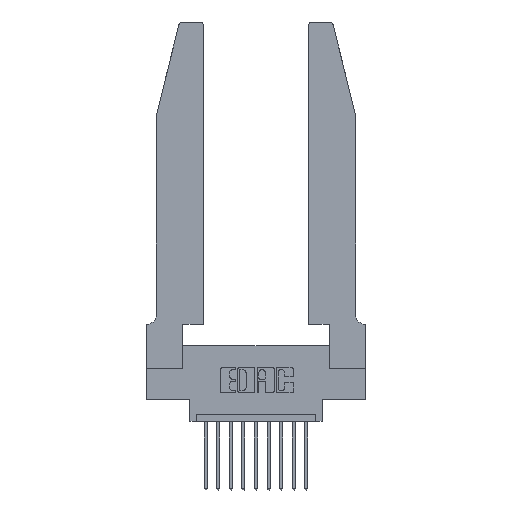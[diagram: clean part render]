
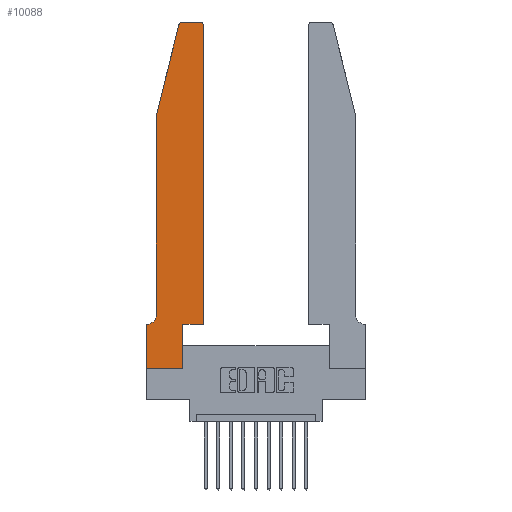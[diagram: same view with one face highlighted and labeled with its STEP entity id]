
A CAD part, top view. The second image highlights one B-rep face of the part: STEP entity #10088.
In plain terms, the highlighted planar face has unit normal (0, 0, 1).
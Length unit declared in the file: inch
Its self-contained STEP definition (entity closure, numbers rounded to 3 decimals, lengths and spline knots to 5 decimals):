
#271 = AXIS2_PLACEMENT_3D ( 'NONE', #14852, #7218, #7381 ) ;
#731 = DIRECTION ( 'NONE',  ( 1., 0., 0. ) ) ;
#881 = ORIENTED_EDGE ( 'NONE', *, *, #12736, .T. ) ;
#1047 = ORIENTED_EDGE ( 'NONE', *, *, #1208, .T. ) ;
#1116 = VECTOR ( 'NONE', #6995, 39.37008 ) ;
#1201 = VECTOR ( 'NONE', #15198, 39.37008 ) ;
#1208 = EDGE_CURVE ( 'NONE', #14253, #4587, #13218, .T. ) ;
#1744 = CARTESIAN_POINT ( 'NONE',  ( 0.0755, 2., 0.37 ) ) ;
#1786 = CARTESIAN_POINT ( 'NONE',  ( 0.2865, 0., 0.37 ) ) ;
#1848 = EDGE_CURVE ( 'NONE', #2867, #7956, #15561, .T. ) ;
#1938 = ORIENTED_EDGE ( 'NONE', *, *, #12678, .T. ) ;
#2620 = CARTESIAN_POINT ( 'NONE',  ( 0.4205, 2.75, 0.37 ) ) ;
#2723 = FACE_OUTER_BOUND ( 'NONE', #6679, .T. ) ;
#2867 = VERTEX_POINT ( 'NONE', #9042 ) ;
#2932 = ORIENTED_EDGE ( 'NONE', *, *, #13490, .T. ) ;
#2975 = LINE ( 'NONE', #7670, #1201 ) ;
#2981 = EDGE_CURVE ( 'NONE', #8498, #5443, #2975, .T. ) ;
#2985 = CARTESIAN_POINT ( 'NONE',  ( 0., 0., 0.37 ) ) ;
#3156 = CARTESIAN_POINT ( 'NONE',  ( 0., 0., 0.37 ) ) ;
#3195 = DIRECTION ( 'NONE',  ( 0., -1., 0. ) ) ;
#3352 = ORIENTED_EDGE ( 'NONE', *, *, #4293, .T. ) ;
#3621 = CARTESIAN_POINT ( 'NONE',  ( 0.2865, 0.35, 0.37 ) ) ;
#3913 = AXIS2_PLACEMENT_3D ( 'NONE', #9033, #8985, #4082 ) ;
#3989 = CARTESIAN_POINT ( 'NONE',  ( 0.2605, 2.75, 0.37 ) ) ;
#4014 = ORIENTED_EDGE ( 'NONE', *, *, #2981, .T. ) ;
#4082 = DIRECTION ( 'NONE',  ( -1., 0., 0. ) ) ;
#4103 = ORIENTED_EDGE ( 'NONE', *, *, #10048, .T. ) ;
#4210 = VECTOR ( 'NONE', #16006, 39.37008 ) ;
#4254 = DIRECTION ( 'NONE',  ( -0.239, -0.971, 0. ) ) ;
#4293 = EDGE_CURVE ( 'NONE', #6805, #8498, #6608, .T. ) ;
#4323 = CARTESIAN_POINT ( 'NONE',  ( 0., 0., 0.37 ) ) ;
#4379 = DIRECTION ( 'NONE',  ( 1., 0., 0. ) ) ;
#4436 = CIRCLE ( 'NONE', #271, 0.03 ) ;
#4440 = VERTEX_POINT ( 'NONE', #13590 ) ;
#4587 = VERTEX_POINT ( 'NONE', #4323 ) ;
#5264 = CIRCLE ( 'NONE', #11125, 0.03 ) ;
#5273 = ORIENTED_EDGE ( 'NONE', *, *, #9063, .T. ) ;
#5336 = EDGE_CURVE ( 'NONE', #7956, #4440, #7933, .T. ) ;
#5428 = VECTOR ( 'NONE', #13722, 39.37008 ) ;
#5443 = VERTEX_POINT ( 'NONE', #14739 ) ;
#5478 = EDGE_CURVE ( 'NONE', #5443, #14149, #4436, .T. ) ;
#5791 = CARTESIAN_POINT ( 'NONE',  ( 0.0755, 2., 0.37 ) ) ;
#6089 = VECTOR ( 'NONE', #4379, 39.37008 ) ;
#6139 = LINE ( 'NONE', #3621, #4210 ) ;
#6383 = CARTESIAN_POINT ( 'NONE',  ( 0.2865, 0.35, 0.37 ) ) ;
#6608 = LINE ( 'NONE', #8435, #12043 ) ;
#6679 = EDGE_LOOP ( 'NONE', ( #2932, #881, #8239, #12461, #5273, #4103, #1047, #1938, #10262, #3352, #4014, #11925 ) ) ;
#6778 = LINE ( 'NONE', #7351, #5428 ) ;
#6805 = VERTEX_POINT ( 'NONE', #6383 ) ;
#6995 = DIRECTION ( 'NONE',  ( 0., -1., 0. ) ) ;
#7107 = VERTEX_POINT ( 'NONE', #1786 ) ;
#7218 = DIRECTION ( 'NONE',  ( 0., 0., 1. ) ) ;
#7230 = VERTEX_POINT ( 'NONE', #11756 ) ;
#7351 = CARTESIAN_POINT ( 'NONE',  ( 0.0755, 0.35, 0.37 ) ) ;
#7381 = DIRECTION ( 'NONE',  ( 1., 0., 0. ) ) ;
#7388 = EDGE_CURVE ( 'NONE', #7107, #6805, #6139, .T. ) ;
#7670 = CARTESIAN_POINT ( 'NONE',  ( 0.4505, 0.35, 0.37 ) ) ;
#7679 = DIRECTION ( 'NONE',  ( -1., 0., 0. ) ) ;
#7772 = VERTEX_POINT ( 'NONE', #9556 ) ;
#7933 = LINE ( 'NONE', #5791, #1116 ) ;
#7956 = VERTEX_POINT ( 'NONE', #10063 ) ;
#8239 = ORIENTED_EDGE ( 'NONE', *, *, #1848, .T. ) ;
#8292 = CARTESIAN_POINT ( 'NONE',  ( 0.4505, 0.35, 0.37 ) ) ;
#8435 = CARTESIAN_POINT ( 'NONE',  ( 0.4505, 0.35, 0.37 ) ) ;
#8498 = VERTEX_POINT ( 'NONE', #8292 ) ;
#8610 = CARTESIAN_POINT ( 'NONE',  ( 0., 0.35, 0.37 ) ) ;
#8985 = DIRECTION ( 'NONE',  ( 0., 0., -1. ) ) ;
#9033 = CARTESIAN_POINT ( 'NONE',  ( 0.0055, 0.42, 0.37 ) ) ;
#9038 = AXIS2_PLACEMENT_3D ( 'NONE', #8610, #12432, #13564 ) ;
#9042 = CARTESIAN_POINT ( 'NONE',  ( 0.25487, 2.72718, 0.37 ) ) ;
#9063 = EDGE_CURVE ( 'NONE', #4440, #7772, #11714, .T. ) ;
#9543 = DIRECTION ( 'NONE',  ( 1., 0., 0. ) ) ;
#9556 = CARTESIAN_POINT ( 'NONE',  ( 0.0055, 0.35, 0.37 ) ) ;
#9936 = VECTOR ( 'NONE', #3195, 39.37008 ) ;
#10048 = EDGE_CURVE ( 'NONE', #7772, #14253, #6778, .T. ) ;
#10063 = CARTESIAN_POINT ( 'NONE',  ( 0.0755, 2., 0.37 ) ) ;
#10088 = ADVANCED_FACE ( 'NONE', ( #2723 ), #13499, .T. ) ;
#10262 = ORIENTED_EDGE ( 'NONE', *, *, #7388, .T. ) ;
#10398 = CARTESIAN_POINT ( 'NONE',  ( 0., 0.35, 0.37 ) ) ;
#10486 = CARTESIAN_POINT ( 'NONE',  ( 0.284, 2.72, 0.37 ) ) ;
#11114 = LINE ( 'NONE', #3989, #12295 ) ;
#11125 = AXIS2_PLACEMENT_3D ( 'NONE', #10486, #15493, #731 ) ;
#11714 = CIRCLE ( 'NONE', #3913, 0.07 ) ;
#11756 = CARTESIAN_POINT ( 'NONE',  ( 0.284, 2.75, 0.37 ) ) ;
#11841 = VECTOR ( 'NONE', #4254, 39.37008 ) ;
#11925 = ORIENTED_EDGE ( 'NONE', *, *, #5478, .T. ) ;
#12043 = VECTOR ( 'NONE', #9543, 39.37008 ) ;
#12295 = VECTOR ( 'NONE', #7679, 39.37008 ) ;
#12432 = DIRECTION ( 'NONE',  ( 0., 0., 1. ) ) ;
#12461 = ORIENTED_EDGE ( 'NONE', *, *, #5336, .T. ) ;
#12678 = EDGE_CURVE ( 'NONE', #4587, #7107, #15390, .T. ) ;
#12736 = EDGE_CURVE ( 'NONE', #7230, #2867, #5264, .T. ) ;
#13218 = LINE ( 'NONE', #2985, #9936 ) ;
#13490 = EDGE_CURVE ( 'NONE', #14149, #7230, #11114, .T. ) ;
#13499 = PLANE ( 'NONE',  #9038 ) ;
#13564 = DIRECTION ( 'NONE',  ( 1., 0., 0. ) ) ;
#13590 = CARTESIAN_POINT ( 'NONE',  ( 0.0755, 0.42, 0.37 ) ) ;
#13722 = DIRECTION ( 'NONE',  ( -1., 0., 0. ) ) ;
#14149 = VERTEX_POINT ( 'NONE', #2620 ) ;
#14253 = VERTEX_POINT ( 'NONE', #10398 ) ;
#14739 = CARTESIAN_POINT ( 'NONE',  ( 0.4505, 2.72, 0.37 ) ) ;
#14852 = CARTESIAN_POINT ( 'NONE',  ( 0.4205, 2.72, 0.37 ) ) ;
#15198 = DIRECTION ( 'NONE',  ( 0., 1., 0. ) ) ;
#15390 = LINE ( 'NONE', #3156, #6089 ) ;
#15493 = DIRECTION ( 'NONE',  ( 0., 0., 1. ) ) ;
#15561 = LINE ( 'NONE', #1744, #11841 ) ;
#16006 = DIRECTION ( 'NONE',  ( 0., 1., 0. ) ) ;
